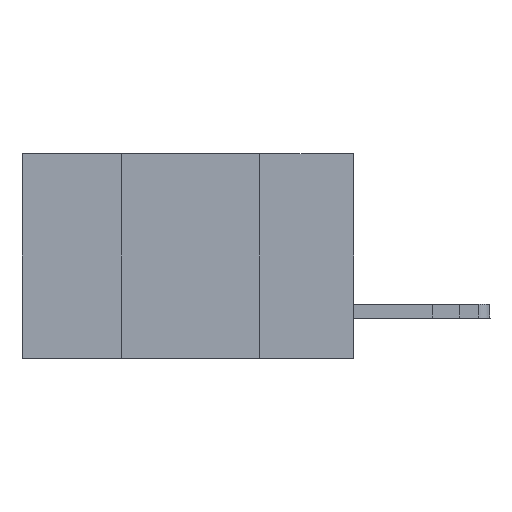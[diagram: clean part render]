
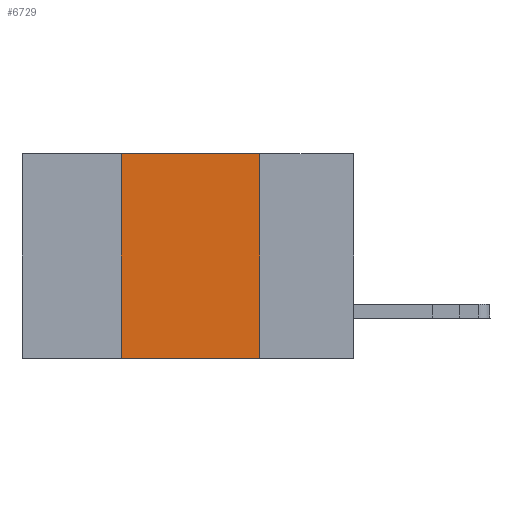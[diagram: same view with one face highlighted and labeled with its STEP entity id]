
A CAD part, left-side view. The second image highlights one B-rep face of the part: STEP entity #6729.
In plain terms, the highlighted planar face has unit normal (-1, 0, 0).
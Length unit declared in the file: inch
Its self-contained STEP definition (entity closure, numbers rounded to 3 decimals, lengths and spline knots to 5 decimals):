
#1945 = FACE_OUTER_BOUND ( 'NONE', #11045, .T. ) ;
#2012 = DIRECTION ( 'NONE',  ( 0., 0., 1. ) ) ;
#3063 = CARTESIAN_POINT ( 'NONE',  ( 0., 0.42, -0.37 ) ) ;
#3674 = AXIS2_PLACEMENT_3D ( 'NONE', #15450, #18963, #13485 ) ;
#3997 = LINE ( 'NONE', #20983, #17517 ) ;
#6729 = ADVANCED_FACE ( 'NONE', ( #1945 ), #11758, .F. ) ;
#7608 = VERTEX_POINT ( 'NONE', #19999 ) ;
#8654 = VECTOR ( 'NONE', #12120, 39.37008 ) ;
#9711 = EDGE_CURVE ( 'NONE', #7608, #16815, #18501, .T. ) ;
#9840 = DIRECTION ( 'NONE',  ( 0., -1., 0. ) ) ;
#9959 = VERTEX_POINT ( 'NONE', #22151 ) ;
#10127 = CARTESIAN_POINT ( 'NONE',  ( 0., 0.6, -0.37 ) ) ;
#10331 = DIRECTION ( 'NONE',  ( 0., 0., -1. ) ) ;
#10401 = CARTESIAN_POINT ( 'NONE',  ( 0., 0.17, 0. ) ) ;
#11045 = EDGE_LOOP ( 'NONE', ( #15840, #21880, #18986, #14592 ) ) ;
#11445 = VECTOR ( 'NONE', #9840, 39.37008 ) ;
#11502 = VERTEX_POINT ( 'NONE', #3063 ) ;
#11758 = PLANE ( 'NONE',  #3674 ) ;
#11943 = LINE ( 'NONE', #10127, #8654 ) ;
#12120 = DIRECTION ( 'NONE',  ( 0., -1., 0. ) ) ;
#13485 = DIRECTION ( 'NONE',  ( 0., 0., -1. ) ) ;
#14592 = ORIENTED_EDGE ( 'NONE', *, *, #21746, .T. ) ;
#15238 = VECTOR ( 'NONE', #10331, 39.37008 ) ;
#15450 = CARTESIAN_POINT ( 'NONE',  ( 0., 0.6, 0. ) ) ;
#15840 = ORIENTED_EDGE ( 'NONE', *, *, #17155, .F. ) ;
#16815 = VERTEX_POINT ( 'NONE', #22318 ) ;
#16991 = CARTESIAN_POINT ( 'NONE',  ( 0., 0.6, 0. ) ) ;
#17155 = EDGE_CURVE ( 'NONE', #16815, #9959, #20131, .T. ) ;
#17517 = VECTOR ( 'NONE', #2012, 39.37008 ) ;
#18501 = LINE ( 'NONE', #16991, #11445 ) ;
#18963 = DIRECTION ( 'NONE',  ( 1., 0., 0. ) ) ;
#18986 = ORIENTED_EDGE ( 'NONE', *, *, #21157, .F. ) ;
#19999 = CARTESIAN_POINT ( 'NONE',  ( 0., 0.42, 0. ) ) ;
#20131 = LINE ( 'NONE', #10401, #15238 ) ;
#20983 = CARTESIAN_POINT ( 'NONE',  ( 0., 0.42, 0. ) ) ;
#21157 = EDGE_CURVE ( 'NONE', #11502, #7608, #3997, .T. ) ;
#21746 = EDGE_CURVE ( 'NONE', #11502, #9959, #11943, .T. ) ;
#21880 = ORIENTED_EDGE ( 'NONE', *, *, #9711, .F. ) ;
#22151 = CARTESIAN_POINT ( 'NONE',  ( 0., 0.17, -0.37 ) ) ;
#22318 = CARTESIAN_POINT ( 'NONE',  ( 0., 0.17, 0. ) ) ;
